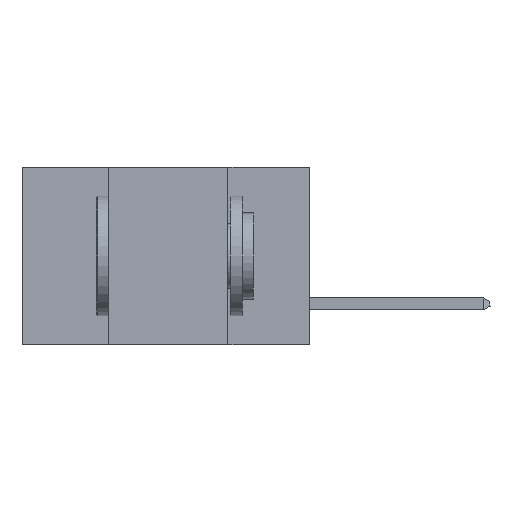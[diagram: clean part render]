
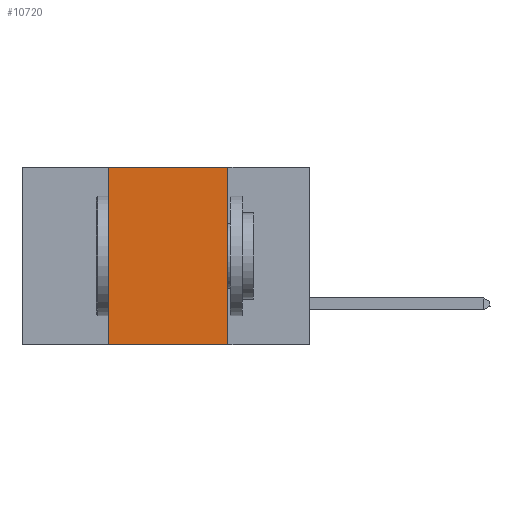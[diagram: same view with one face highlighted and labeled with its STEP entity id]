
A CAD part, left-side view. The second image highlights one B-rep face of the part: STEP entity #10720.
In plain terms, the highlighted planar face has unit normal (-1, 0, 0).
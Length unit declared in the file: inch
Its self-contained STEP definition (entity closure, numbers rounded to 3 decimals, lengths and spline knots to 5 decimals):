
#610 = VERTEX_POINT ( 'NONE', #6283 ) ;
#829 = LINE ( 'NONE', #12869, #5117 ) ;
#859 = ORIENTED_EDGE ( 'NONE', *, *, #11186, .T. ) ;
#875 = ORIENTED_EDGE ( 'NONE', *, *, #5578, .F. ) ;
#1045 = LINE ( 'NONE', #4782, #11833 ) ;
#1491 = DIRECTION ( 'NONE',  ( 0., 0., -1. ) ) ;
#1655 = DIRECTION ( 'NONE',  ( 0., 0., -1. ) ) ;
#2411 = CARTESIAN_POINT ( 'NONE',  ( 0., 0.6, 0. ) ) ;
#2732 = FACE_OUTER_BOUND ( 'NONE', #8606, .T. ) ;
#2802 = LINE ( 'NONE', #8752, #5730 ) ;
#3022 = CARTESIAN_POINT ( 'NONE',  ( 0., 0.17, -0.37 ) ) ;
#4782 = CARTESIAN_POINT ( 'NONE',  ( 0., 0.42, 0. ) ) ;
#4911 = VERTEX_POINT ( 'NONE', #3022 ) ;
#4961 = CARTESIAN_POINT ( 'NONE',  ( 0., 0.17, 0. ) ) ;
#5117 = VECTOR ( 'NONE', #12970, 39.37008 ) ;
#5578 = EDGE_CURVE ( 'NONE', #10882, #13460, #1045, .T. ) ;
#5730 = VECTOR ( 'NONE', #13269, 39.37008 ) ;
#6283 = CARTESIAN_POINT ( 'NONE',  ( 0., 0.17, 0. ) ) ;
#6960 = DIRECTION ( 'NONE',  ( 0., 0., 1. ) ) ;
#8128 = DIRECTION ( 'NONE',  ( 1., 0., 0. ) ) ;
#8409 = ORIENTED_EDGE ( 'NONE', *, *, #14457, .F. ) ;
#8606 = EDGE_LOOP ( 'NONE', ( #8409, #13497, #875, #859 ) ) ;
#8752 = CARTESIAN_POINT ( 'NONE',  ( 0., 0.6, 0. ) ) ;
#9093 = PLANE ( 'NONE',  #11545 ) ;
#9150 = EDGE_CURVE ( 'NONE', #13460, #610, #2802, .T. ) ;
#10248 = CARTESIAN_POINT ( 'NONE',  ( 0., 0.42, 0. ) ) ;
#10720 = ADVANCED_FACE ( 'NONE', ( #2732 ), #9093, .F. ) ;
#10882 = VERTEX_POINT ( 'NONE', #13511 ) ;
#10973 = LINE ( 'NONE', #4961, #11136 ) ;
#11136 = VECTOR ( 'NONE', #1655, 39.37008 ) ;
#11186 = EDGE_CURVE ( 'NONE', #10882, #4911, #829, .T. ) ;
#11545 = AXIS2_PLACEMENT_3D ( 'NONE', #2411, #8128, #1491 ) ;
#11833 = VECTOR ( 'NONE', #6960, 39.37008 ) ;
#12869 = CARTESIAN_POINT ( 'NONE',  ( 0., 0.6, -0.37 ) ) ;
#12970 = DIRECTION ( 'NONE',  ( 0., -1., 0. ) ) ;
#13269 = DIRECTION ( 'NONE',  ( 0., -1., 0. ) ) ;
#13460 = VERTEX_POINT ( 'NONE', #10248 ) ;
#13497 = ORIENTED_EDGE ( 'NONE', *, *, #9150, .F. ) ;
#13511 = CARTESIAN_POINT ( 'NONE',  ( 0., 0.42, -0.37 ) ) ;
#14457 = EDGE_CURVE ( 'NONE', #610, #4911, #10973, .T. ) ;
